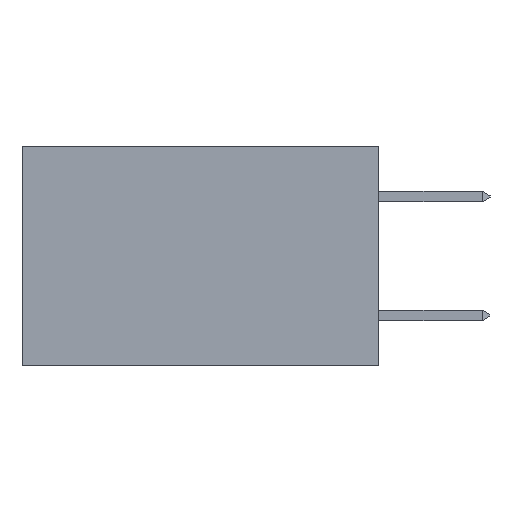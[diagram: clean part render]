
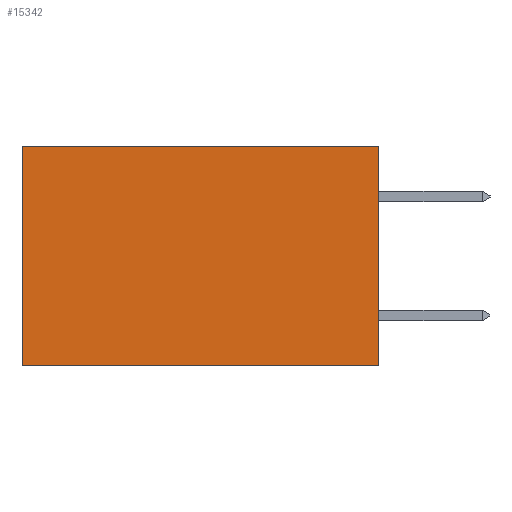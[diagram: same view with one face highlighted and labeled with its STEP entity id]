
A CAD part, left-side view. The second image highlights one B-rep face of the part: STEP entity #15342.
In plain terms, the highlighted planar face has unit normal (-1, 0, 0).
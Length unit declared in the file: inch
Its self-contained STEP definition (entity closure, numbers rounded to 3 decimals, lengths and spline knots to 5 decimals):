
#202 = EDGE_CURVE ( 'NONE', #2425, #4479, #12072, .T. ) ;
#391 = VERTEX_POINT ( 'NONE', #4305 ) ;
#676 = CARTESIAN_POINT ( 'NONE',  ( 0.2615, 0., -0.37 ) ) ;
#936 = DIRECTION ( 'NONE',  ( 0., 0., -1. ) ) ;
#1027 = VECTOR ( 'NONE', #21648, 39.37008 ) ;
#2425 = VERTEX_POINT ( 'NONE', #676 ) ;
#3665 = ORIENTED_EDGE ( 'NONE', *, *, #17734, .T. ) ;
#3742 = DIRECTION ( 'NONE',  ( 0., 1., 0. ) ) ;
#3880 = CARTESIAN_POINT ( 'NONE',  ( 0.2615, 0.6, -0.37 ) ) ;
#4305 = CARTESIAN_POINT ( 'NONE',  ( 0.2615, 0.6, 0. ) ) ;
#4384 = EDGE_CURVE ( 'NONE', #6259, #2425, #19787, .T. ) ;
#4479 = VERTEX_POINT ( 'NONE', #3880 ) ;
#4491 = CARTESIAN_POINT ( 'NONE',  ( 0.2615, 0., -0.37 ) ) ;
#5293 = ORIENTED_EDGE ( 'NONE', *, *, #8839, .T. ) ;
#5532 = LINE ( 'NONE', #21191, #14335 ) ;
#6259 = VERTEX_POINT ( 'NONE', #18557 ) ;
#6846 = VECTOR ( 'NONE', #12021, 39.37008 ) ;
#6904 = VECTOR ( 'NONE', #20728, 39.37008 ) ;
#6978 = AXIS2_PLACEMENT_3D ( 'NONE', #4491, #11613, #936 ) ;
#8491 = CARTESIAN_POINT ( 'NONE',  ( 0.2615, 0., -0.37 ) ) ;
#8839 = EDGE_CURVE ( 'NONE', #391, #4479, #11571, .T. ) ;
#9908 = ORIENTED_EDGE ( 'NONE', *, *, #202, .F. ) ;
#11571 = LINE ( 'NONE', #11987, #6904 ) ;
#11613 = DIRECTION ( 'NONE',  ( 1., 0., 0. ) ) ;
#11987 = CARTESIAN_POINT ( 'NONE',  ( 0.2615, 0.6, -0.37 ) ) ;
#12021 = DIRECTION ( 'NONE',  ( 0., 1., 0. ) ) ;
#12072 = LINE ( 'NONE', #8491, #6846 ) ;
#14335 = VECTOR ( 'NONE', #3742, 39.37008 ) ;
#15342 = ADVANCED_FACE ( 'NONE', ( #21222 ), #22000, .F. ) ;
#17651 = ORIENTED_EDGE ( 'NONE', *, *, #4384, .F. ) ;
#17734 = EDGE_CURVE ( 'NONE', #6259, #391, #5532, .T. ) ;
#18557 = CARTESIAN_POINT ( 'NONE',  ( 0.2615, 0., 0. ) ) ;
#18737 = EDGE_LOOP ( 'NONE', ( #5293, #9908, #17651, #3665 ) ) ;
#19787 = LINE ( 'NONE', #19832, #1027 ) ;
#19832 = CARTESIAN_POINT ( 'NONE',  ( 0.2615, 0., -0.37 ) ) ;
#20728 = DIRECTION ( 'NONE',  ( 0., 0., -1. ) ) ;
#21191 = CARTESIAN_POINT ( 'NONE',  ( 0.2615, 0., 0. ) ) ;
#21222 = FACE_OUTER_BOUND ( 'NONE', #18737, .T. ) ;
#21648 = DIRECTION ( 'NONE',  ( 0., 0., -1. ) ) ;
#22000 = PLANE ( 'NONE',  #6978 ) ;
